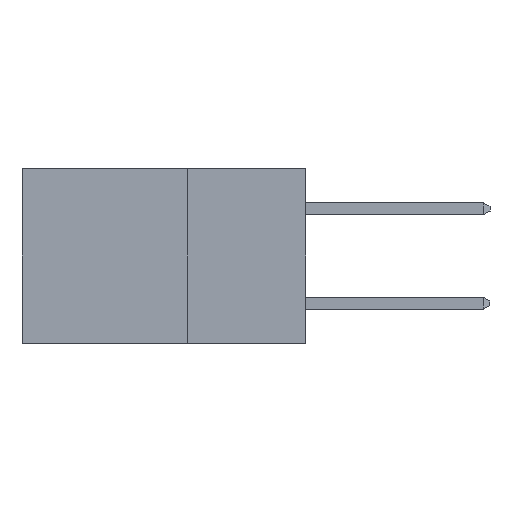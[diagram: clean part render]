
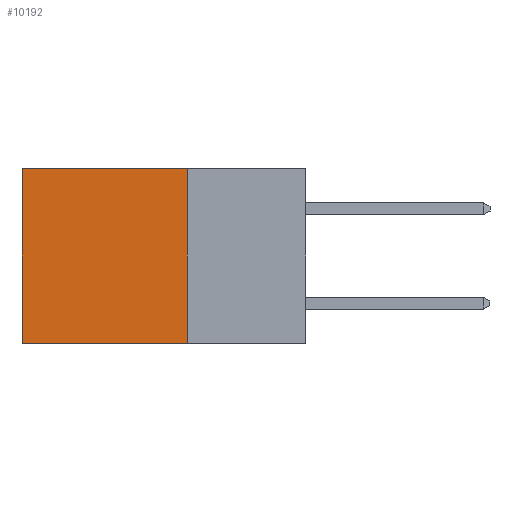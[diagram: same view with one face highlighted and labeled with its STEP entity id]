
A CAD part, left-side view. The second image highlights one B-rep face of the part: STEP entity #10192.
In plain terms, the highlighted planar face has unit normal (-1, 0, 0).
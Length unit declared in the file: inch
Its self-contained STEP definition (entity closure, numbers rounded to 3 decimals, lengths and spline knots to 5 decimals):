
#21 = LINE ( 'NONE', #4284, #7512 ) ;
#122 = DIRECTION ( 'NONE',  ( 1., 0., 0. ) ) ;
#705 = VERTEX_POINT ( 'NONE', #9793 ) ;
#1441 = EDGE_CURVE ( 'NONE', #8338, #11268, #12210, .T. ) ;
#1980 = VECTOR ( 'NONE', #5408, 39.37008 ) ;
#2004 = CARTESIAN_POINT ( 'NONE',  ( 0.298, 0.25, -0.37 ) ) ;
#2297 = VERTEX_POINT ( 'NONE', #2004 ) ;
#2433 = EDGE_CURVE ( 'NONE', #8338, #2297, #21, .T. ) ;
#2520 = LINE ( 'NONE', #2944, #5426 ) ;
#2944 = CARTESIAN_POINT ( 'NONE',  ( 0.298, 0.6, 0. ) ) ;
#3609 = EDGE_LOOP ( 'NONE', ( #11847, #12370, #11461, #9410 ) ) ;
#4284 = CARTESIAN_POINT ( 'NONE',  ( 0.298, 0.25, 0. ) ) ;
#4564 = DIRECTION ( 'NONE',  ( 0., 1., 0. ) ) ;
#4736 = CARTESIAN_POINT ( 'NONE',  ( 0.298, 0.6, 0. ) ) ;
#5408 = DIRECTION ( 'NONE',  ( 0., 1., 0. ) ) ;
#5426 = VECTOR ( 'NONE', #8556, 39.37008 ) ;
#5652 = EDGE_CURVE ( 'NONE', #2297, #705, #8475, .T. ) ;
#5873 = CARTESIAN_POINT ( 'NONE',  ( 0.298, 0.25, -0.37 ) ) ;
#6276 = VECTOR ( 'NONE', #4564, 39.37008 ) ;
#6977 = DIRECTION ( 'NONE',  ( 0., 0., -1. ) ) ;
#7512 = VECTOR ( 'NONE', #7690, 39.37008 ) ;
#7690 = DIRECTION ( 'NONE',  ( 0., 0., -1. ) ) ;
#7899 = PLANE ( 'NONE',  #8926 ) ;
#8328 = CARTESIAN_POINT ( 'NONE',  ( 0.298, 0.25, 0. ) ) ;
#8338 = VERTEX_POINT ( 'NONE', #10816 ) ;
#8475 = LINE ( 'NONE', #5873, #6276 ) ;
#8556 = DIRECTION ( 'NONE',  ( 0., 0., -1. ) ) ;
#8926 = AXIS2_PLACEMENT_3D ( 'NONE', #10814, #122, #6977 ) ;
#9410 = ORIENTED_EDGE ( 'NONE', *, *, #1441, .T. ) ;
#9793 = CARTESIAN_POINT ( 'NONE',  ( 0.298, 0.6, -0.37 ) ) ;
#9964 = EDGE_CURVE ( 'NONE', #11268, #705, #2520, .T. ) ;
#10192 = ADVANCED_FACE ( 'NONE', ( #12501 ), #7899, .F. ) ;
#10814 = CARTESIAN_POINT ( 'NONE',  ( 0.298, 0.25, 0. ) ) ;
#10816 = CARTESIAN_POINT ( 'NONE',  ( 0.298, 0.25, 0. ) ) ;
#11268 = VERTEX_POINT ( 'NONE', #4736 ) ;
#11461 = ORIENTED_EDGE ( 'NONE', *, *, #2433, .F. ) ;
#11847 = ORIENTED_EDGE ( 'NONE', *, *, #9964, .T. ) ;
#12210 = LINE ( 'NONE', #8328, #1980 ) ;
#12370 = ORIENTED_EDGE ( 'NONE', *, *, #5652, .F. ) ;
#12501 = FACE_OUTER_BOUND ( 'NONE', #3609, .T. ) ;
